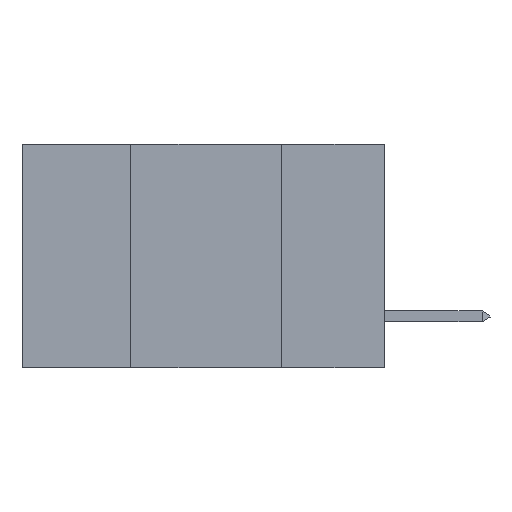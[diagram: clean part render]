
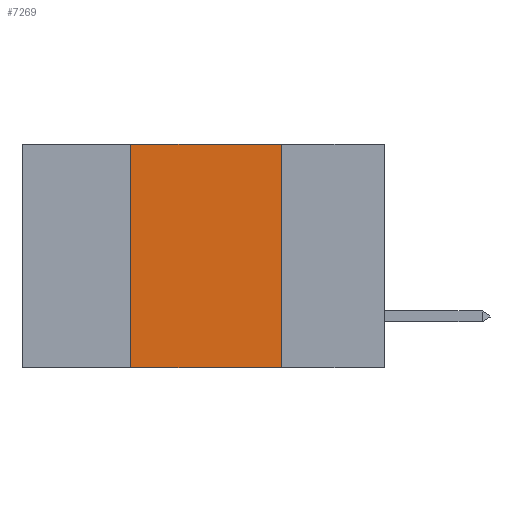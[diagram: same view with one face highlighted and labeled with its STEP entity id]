
A CAD part, left-side view. The second image highlights one B-rep face of the part: STEP entity #7269.
In plain terms, the highlighted planar face has unit normal (-1, 0, 0).
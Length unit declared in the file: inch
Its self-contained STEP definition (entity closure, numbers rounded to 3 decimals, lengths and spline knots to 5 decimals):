
#864 = DIRECTION ( 'NONE',  ( 0., 0., -1. ) ) ;
#1415 = CARTESIAN_POINT ( 'NONE',  ( 0., 0.6, 0. ) ) ;
#2308 = FACE_OUTER_BOUND ( 'NONE', #17365, .T. ) ;
#2857 = CARTESIAN_POINT ( 'NONE',  ( 0., 0.42, 0. ) ) ;
#4160 = AXIS2_PLACEMENT_3D ( 'NONE', #1415, #34333, #864 ) ;
#4278 = ORIENTED_EDGE ( 'NONE', *, *, #38112, .F. ) ;
#4972 = LINE ( 'NONE', #15136, #12012 ) ;
#6832 = EDGE_CURVE ( 'NONE', #28531, #37380, #37324, .T. ) ;
#7269 = ADVANCED_FACE ( 'NONE', ( #2308 ), #9997, .F. ) ;
#7457 = EDGE_CURVE ( 'NONE', #28966, #28531, #14103, .T. ) ;
#7541 = VECTOR ( 'NONE', #31046, 39.37008 ) ;
#9586 = DIRECTION ( 'NONE',  ( 0., 0., 1. ) ) ;
#9997 = PLANE ( 'NONE',  #4160 ) ;
#10841 = LINE ( 'NONE', #34129, #7541 ) ;
#11396 = VERTEX_POINT ( 'NONE', #25442 ) ;
#12012 = VECTOR ( 'NONE', #12074, 39.37008 ) ;
#12074 = DIRECTION ( 'NONE',  ( 0., -1., 0. ) ) ;
#12421 = ORIENTED_EDGE ( 'NONE', *, *, #6832, .F. ) ;
#12690 = VECTOR ( 'NONE', #27398, 39.37008 ) ;
#14103 = LINE ( 'NONE', #36977, #35409 ) ;
#15136 = CARTESIAN_POINT ( 'NONE',  ( 0., 0.6, -0.37 ) ) ;
#17116 = CARTESIAN_POINT ( 'NONE',  ( 0., 0.17, 0. ) ) ;
#17365 = EDGE_LOOP ( 'NONE', ( #4278, #12421, #21141, #32075 ) ) ;
#21141 = ORIENTED_EDGE ( 'NONE', *, *, #7457, .F. ) ;
#23403 = CARTESIAN_POINT ( 'NONE',  ( 0., 0.42, -0.37 ) ) ;
#25442 = CARTESIAN_POINT ( 'NONE',  ( 0., 0.17, -0.37 ) ) ;
#27398 = DIRECTION ( 'NONE',  ( 0., -1., 0. ) ) ;
#28531 = VERTEX_POINT ( 'NONE', #2857 ) ;
#28966 = VERTEX_POINT ( 'NONE', #23403 ) ;
#31046 = DIRECTION ( 'NONE',  ( 0., 0., -1. ) ) ;
#32075 = ORIENTED_EDGE ( 'NONE', *, *, #36971, .T. ) ;
#33755 = CARTESIAN_POINT ( 'NONE',  ( 0., 0.6, 0. ) ) ;
#34129 = CARTESIAN_POINT ( 'NONE',  ( 0., 0.17, 0. ) ) ;
#34333 = DIRECTION ( 'NONE',  ( 1., 0., 0. ) ) ;
#35409 = VECTOR ( 'NONE', #9586, 39.37008 ) ;
#36971 = EDGE_CURVE ( 'NONE', #28966, #11396, #4972, .T. ) ;
#36977 = CARTESIAN_POINT ( 'NONE',  ( 0., 0.42, 0. ) ) ;
#37324 = LINE ( 'NONE', #33755, #12690 ) ;
#37380 = VERTEX_POINT ( 'NONE', #17116 ) ;
#38112 = EDGE_CURVE ( 'NONE', #37380, #11396, #10841, .T. ) ;
